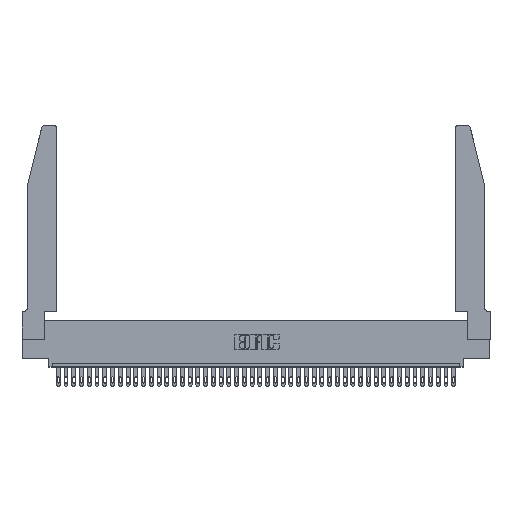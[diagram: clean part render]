
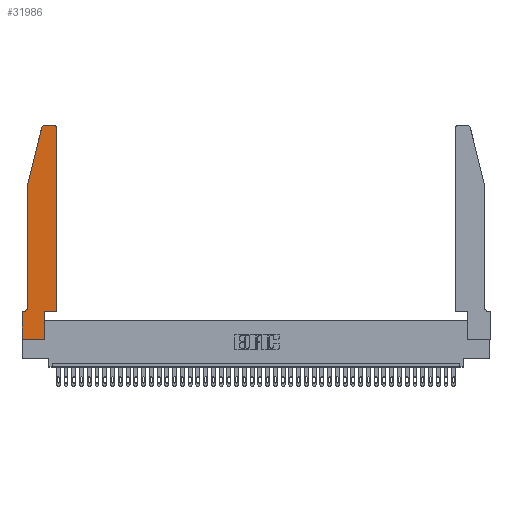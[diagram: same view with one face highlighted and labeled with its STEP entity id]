
A CAD part, top view. The second image highlights one B-rep face of the part: STEP entity #31986.
In plain terms, the highlighted planar face has unit normal (0, 0, 1).
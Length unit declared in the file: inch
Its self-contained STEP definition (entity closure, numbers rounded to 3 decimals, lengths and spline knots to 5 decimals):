
#274 = LINE ( 'NONE', #14800, #34219 ) ;
#974 = DIRECTION ( 'NONE',  ( 1., 0., 0. ) ) ;
#1398 = ORIENTED_EDGE ( 'NONE', *, *, #5571, .T. ) ;
#1437 = ORIENTED_EDGE ( 'NONE', *, *, #16823, .T. ) ;
#1853 = ORIENTED_EDGE ( 'NONE', *, *, #6244, .T. ) ;
#2376 = DIRECTION ( 'NONE',  ( 0., -1., 0. ) ) ;
#2595 = DIRECTION ( 'NONE',  ( -1., 0., 0. ) ) ;
#3235 = CARTESIAN_POINT ( 'NONE',  ( 0.2865, 0.35, 0.37 ) ) ;
#3677 = CARTESIAN_POINT ( 'NONE',  ( 0.0755, 2., 0.37 ) ) ;
#4375 = ORIENTED_EDGE ( 'NONE', *, *, #27251, .T. ) ;
#5109 = ORIENTED_EDGE ( 'NONE', *, *, #33424, .T. ) ;
#5498 = DIRECTION ( 'NONE',  ( -1., 0., 0. ) ) ;
#5571 = EDGE_CURVE ( 'NONE', #17211, #21383, #274, .T. ) ;
#5659 = CARTESIAN_POINT ( 'NONE',  ( 0.2865, 0., 0.37 ) ) ;
#5735 = CARTESIAN_POINT ( 'NONE',  ( 0., 0., 0.37 ) ) ;
#6244 = EDGE_CURVE ( 'NONE', #26297, #17211, #31598, .T. ) ;
#6857 = CARTESIAN_POINT ( 'NONE',  ( 0.4205, 2.72, 0.37 ) ) ;
#7062 = CARTESIAN_POINT ( 'NONE',  ( 0.2865, 0.35, 0.37 ) ) ;
#7142 = ORIENTED_EDGE ( 'NONE', *, *, #24951, .T. ) ;
#7482 = PLANE ( 'NONE',  #29520 ) ;
#8231 = VECTOR ( 'NONE', #16406, 39.37008 ) ;
#8804 = FACE_OUTER_BOUND ( 'NONE', #13409, .T. ) ;
#8899 = VECTOR ( 'NONE', #2595, 39.37008 ) ;
#9252 = VECTOR ( 'NONE', #5498, 39.37008 ) ;
#9292 = CARTESIAN_POINT ( 'NONE',  ( 0.4205, 2.75, 0.37 ) ) ;
#9724 = CIRCLE ( 'NONE', #21274, 0.03 ) ;
#10539 = CARTESIAN_POINT ( 'NONE',  ( 0., 0.35, 0.37 ) ) ;
#10828 = EDGE_CURVE ( 'NONE', #38027, #26297, #42256, .T. ) ;
#11123 = VERTEX_POINT ( 'NONE', #3677 ) ;
#11507 = VECTOR ( 'NONE', #18114, 39.37008 ) ;
#11961 = VERTEX_POINT ( 'NONE', #42133 ) ;
#13409 = EDGE_LOOP ( 'NONE', ( #34323, #38699, #34639, #37807, #7142, #42346, #5109, #26365, #1853, #1398, #4375, #1437 ) ) ;
#13604 = AXIS2_PLACEMENT_3D ( 'NONE', #30766, #14421, #40695 ) ;
#13795 = DIRECTION ( 'NONE',  ( 0., 0., 1. ) ) ;
#13803 = VERTEX_POINT ( 'NONE', #39964 ) ;
#13907 = CARTESIAN_POINT ( 'NONE',  ( 0.0055, 0.42, 0.37 ) ) ;
#14389 = LINE ( 'NONE', #39238, #8231 ) ;
#14421 = DIRECTION ( 'NONE',  ( 0., 0., 1. ) ) ;
#14506 = VECTOR ( 'NONE', #2376, 39.37008 ) ;
#14800 = CARTESIAN_POINT ( 'NONE',  ( 0.4505, 0.35, 0.37 ) ) ;
#15074 = DIRECTION ( 'NONE',  ( 1., 0., 0. ) ) ;
#15121 = CARTESIAN_POINT ( 'NONE',  ( 0.4505, 0.35, 0.37 ) ) ;
#15528 = CARTESIAN_POINT ( 'NONE',  ( 0.2605, 2.75, 0.37 ) ) ;
#15582 = CIRCLE ( 'NONE', #16149, 0.07 ) ;
#15899 = VERTEX_POINT ( 'NONE', #9292 ) ;
#16149 = AXIS2_PLACEMENT_3D ( 'NONE', #13907, #33861, #24271 ) ;
#16406 = DIRECTION ( 'NONE',  ( 0., -1., 0. ) ) ;
#16823 = EDGE_CURVE ( 'NONE', #18665, #15899, #9724, .T. ) ;
#16955 = DIRECTION ( 'NONE',  ( 0., 1., 0. ) ) ;
#17211 = VERTEX_POINT ( 'NONE', #7062 ) ;
#18114 = DIRECTION ( 'NONE',  ( -0.239, -0.971, 0. ) ) ;
#18665 = VERTEX_POINT ( 'NONE', #39302 ) ;
#19698 = LINE ( 'NONE', #22288, #8899 ) ;
#20230 = LINE ( 'NONE', #24414, #11507 ) ;
#20324 = VECTOR ( 'NONE', #36249, 39.37008 ) ;
#21274 = AXIS2_PLACEMENT_3D ( 'NONE', #6857, #42376, #32585 ) ;
#21383 = VERTEX_POINT ( 'NONE', #15121 ) ;
#22008 = EDGE_CURVE ( 'NONE', #32436, #11123, #20230, .T. ) ;
#22071 = EDGE_CURVE ( 'NONE', #29358, #32436, #22824, .T. ) ;
#22288 = CARTESIAN_POINT ( 'NONE',  ( 0.0755, 0.35, 0.37 ) ) ;
#22824 = CIRCLE ( 'NONE', #13604, 0.03 ) ;
#23168 = CARTESIAN_POINT ( 'NONE',  ( 0.284, 2.75, 0.37 ) ) ;
#24271 = DIRECTION ( 'NONE',  ( -1., 0., 0. ) ) ;
#24414 = CARTESIAN_POINT ( 'NONE',  ( 0.0755, 2., 0.37 ) ) ;
#24951 = EDGE_CURVE ( 'NONE', #11961, #13803, #15582, .T. ) ;
#25144 = VECTOR ( 'NONE', #16955, 39.37008 ) ;
#25675 = CARTESIAN_POINT ( 'NONE',  ( 0.0755, 2., 0.37 ) ) ;
#26030 = CARTESIAN_POINT ( 'NONE',  ( 0.25487, 2.72718, 0.37 ) ) ;
#26297 = VERTEX_POINT ( 'NONE', #5659 ) ;
#26365 = ORIENTED_EDGE ( 'NONE', *, *, #10828, .T. ) ;
#26679 = EDGE_CURVE ( 'NONE', #15899, #29358, #34393, .T. ) ;
#27045 = VERTEX_POINT ( 'NONE', #10539 ) ;
#27251 = EDGE_CURVE ( 'NONE', #21383, #18665, #39481, .T. ) ;
#29358 = VERTEX_POINT ( 'NONE', #23168 ) ;
#29520 = AXIS2_PLACEMENT_3D ( 'NONE', #30418, #13795, #974 ) ;
#30418 = CARTESIAN_POINT ( 'NONE',  ( 0., 0.35, 0.37 ) ) ;
#30766 = CARTESIAN_POINT ( 'NONE',  ( 0.284, 2.72, 0.37 ) ) ;
#31434 = EDGE_CURVE ( 'NONE', #11123, #11961, #37613, .T. ) ;
#31598 = LINE ( 'NONE', #3235, #20324 ) ;
#31986 = ADVANCED_FACE ( 'NONE', ( #8804 ), #7482, .T. ) ;
#32063 = CARTESIAN_POINT ( 'NONE',  ( 0., 0., 0.37 ) ) ;
#32436 = VERTEX_POINT ( 'NONE', #26030 ) ;
#32585 = DIRECTION ( 'NONE',  ( 1., 0., 0. ) ) ;
#32953 = VECTOR ( 'NONE', #38615, 39.37008 ) ;
#33424 = EDGE_CURVE ( 'NONE', #27045, #38027, #14389, .T. ) ;
#33861 = DIRECTION ( 'NONE',  ( 0., 0., -1. ) ) ;
#34219 = VECTOR ( 'NONE', #15074, 39.37008 ) ;
#34323 = ORIENTED_EDGE ( 'NONE', *, *, #26679, .T. ) ;
#34393 = LINE ( 'NONE', #15528, #9252 ) ;
#34639 = ORIENTED_EDGE ( 'NONE', *, *, #22008, .T. ) ;
#36249 = DIRECTION ( 'NONE',  ( 0., 1., 0. ) ) ;
#36333 = CARTESIAN_POINT ( 'NONE',  ( 0.4505, 0.35, 0.37 ) ) ;
#37613 = LINE ( 'NONE', #25675, #14506 ) ;
#37807 = ORIENTED_EDGE ( 'NONE', *, *, #31434, .T. ) ;
#38027 = VERTEX_POINT ( 'NONE', #32063 ) ;
#38615 = DIRECTION ( 'NONE',  ( 1., 0., 0. ) ) ;
#38699 = ORIENTED_EDGE ( 'NONE', *, *, #22071, .T. ) ;
#39238 = CARTESIAN_POINT ( 'NONE',  ( 0., 0., 0.37 ) ) ;
#39302 = CARTESIAN_POINT ( 'NONE',  ( 0.4505, 2.72, 0.37 ) ) ;
#39481 = LINE ( 'NONE', #36333, #25144 ) ;
#39964 = CARTESIAN_POINT ( 'NONE',  ( 0.0055, 0.35, 0.37 ) ) ;
#40695 = DIRECTION ( 'NONE',  ( 1., 0., 0. ) ) ;
#41765 = EDGE_CURVE ( 'NONE', #13803, #27045, #19698, .T. ) ;
#42133 = CARTESIAN_POINT ( 'NONE',  ( 0.0755, 0.42, 0.37 ) ) ;
#42256 = LINE ( 'NONE', #5735, #32953 ) ;
#42346 = ORIENTED_EDGE ( 'NONE', *, *, #41765, .T. ) ;
#42376 = DIRECTION ( 'NONE',  ( 0., 0., 1. ) ) ;
